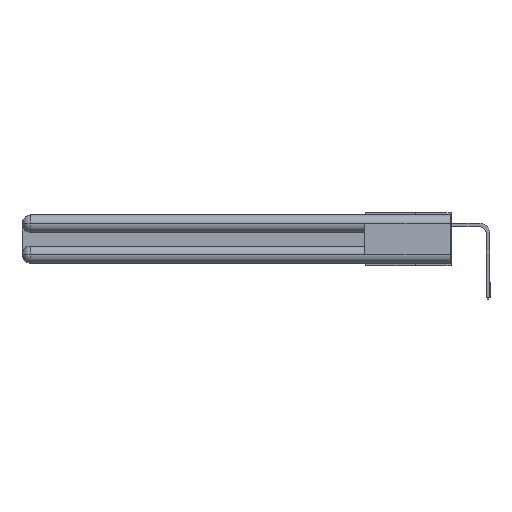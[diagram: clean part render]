
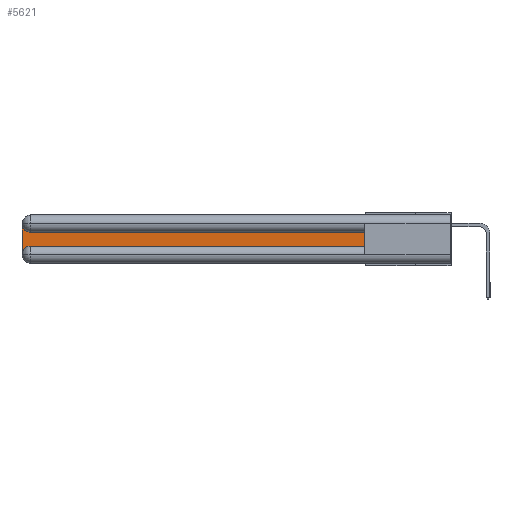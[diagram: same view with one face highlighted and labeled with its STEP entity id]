
A CAD part, left-side view. The second image highlights one B-rep face of the part: STEP entity #5621.
In plain terms, the highlighted planar face has unit normal (-1, 0, 0).
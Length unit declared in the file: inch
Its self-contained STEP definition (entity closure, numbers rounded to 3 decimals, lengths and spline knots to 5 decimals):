
#64 = LINE ( 'NONE', #15927, #16240 ) ;
#335 = CARTESIAN_POINT ( 'NONE',  ( 0.075, 0.6, -0.2175 ) ) ;
#463 = CARTESIAN_POINT ( 'NONE',  ( 0.075, 2.94, -0.2775 ) ) ;
#1160 = VECTOR ( 'NONE', #6062, 39.37008 ) ;
#1681 = CARTESIAN_POINT ( 'NONE',  ( 0.075, 2.94, -0.1225 ) ) ;
#4650 = AXIS2_PLACEMENT_3D ( 'NONE', #8963, #23938, #19724 ) ;
#4861 = VERTEX_POINT ( 'NONE', #23996 ) ;
#4953 = ORIENTED_EDGE ( 'NONE', *, *, #12622, .T. ) ;
#5380 = DIRECTION ( 'NONE',  ( 0., 1., 0. ) ) ;
#5621 = ADVANCED_FACE ( 'NONE', ( #23289 ), #14612, .F. ) ;
#5836 = VECTOR ( 'NONE', #11430, 39.37008 ) ;
#6042 = DIRECTION ( 'NONE',  ( 1., 0., 0. ) ) ;
#6062 = DIRECTION ( 'NONE',  ( 0., 0., 1. ) ) ;
#6643 = EDGE_CURVE ( 'NONE', #27674, #13125, #64, .T. ) ;
#6910 = ORIENTED_EDGE ( 'NONE', *, *, #27615, .T. ) ;
#7510 = ORIENTED_EDGE ( 'NONE', *, *, #6643, .T. ) ;
#8207 = AXIS2_PLACEMENT_3D ( 'NONE', #463, #11471, #17662 ) ;
#8359 = CIRCLE ( 'NONE', #8207, 0.06 ) ;
#8844 = CIRCLE ( 'NONE', #4650, 0.06 ) ;
#8963 = CARTESIAN_POINT ( 'NONE',  ( 0.075, 2.94, -0.0625 ) ) ;
#11143 = CARTESIAN_POINT ( 'NONE',  ( 0.075, 0.6, -0.1225 ) ) ;
#11430 = DIRECTION ( 'NONE',  ( 0., -1., 0. ) ) ;
#11471 = DIRECTION ( 'NONE',  ( 1., 0., 0. ) ) ;
#12327 = ORIENTED_EDGE ( 'NONE', *, *, #13479, .T. ) ;
#12622 = EDGE_CURVE ( 'NONE', #26845, #27674, #16632, .T. ) ;
#13125 = VERTEX_POINT ( 'NONE', #1681 ) ;
#13479 = EDGE_CURVE ( 'NONE', #13125, #24342, #8844, .T. ) ;
#14219 = CARTESIAN_POINT ( 'NONE',  ( 0.075, 3., -0.0625 ) ) ;
#14586 = CARTESIAN_POINT ( 'NONE',  ( 0.075, 2.94, -0.2175 ) ) ;
#14612 = PLANE ( 'NONE',  #21056 ) ;
#14716 = VECTOR ( 'NONE', #23486, 39.37008 ) ;
#14966 = CARTESIAN_POINT ( 'NONE',  ( 0.075, 3., -0.1225 ) ) ;
#15616 = LINE ( 'NONE', #335, #5836 ) ;
#15674 = CARTESIAN_POINT ( 'NONE',  ( 0.075, 0.6, -0.2175 ) ) ;
#15927 = CARTESIAN_POINT ( 'NONE',  ( 0.075, 0.6, -0.1225 ) ) ;
#16240 = VECTOR ( 'NONE', #5380, 39.37008 ) ;
#16632 = LINE ( 'NONE', #23283, #1160 ) ;
#17538 = ORIENTED_EDGE ( 'NONE', *, *, #25268, .T. ) ;
#17662 = DIRECTION ( 'NONE',  ( 0., 0., -1. ) ) ;
#19724 = DIRECTION ( 'NONE',  ( 0., 0., -1. ) ) ;
#20723 = LINE ( 'NONE', #25642, #14716 ) ;
#20839 = EDGE_CURVE ( 'NONE', #4861, #24428, #8359, .T. ) ;
#21043 = DIRECTION ( 'NONE',  ( 0., 0., -1. ) ) ;
#21056 = AXIS2_PLACEMENT_3D ( 'NONE', #14966, #6042, #21043 ) ;
#23283 = CARTESIAN_POINT ( 'NONE',  ( 0.075, 0.6, -0.2175 ) ) ;
#23289 = FACE_OUTER_BOUND ( 'NONE', #26970, .T. ) ;
#23486 = DIRECTION ( 'NONE',  ( 0., 0., -1. ) ) ;
#23938 = DIRECTION ( 'NONE',  ( 1., 0., 0. ) ) ;
#23996 = CARTESIAN_POINT ( 'NONE',  ( 0.075, 3., -0.2775 ) ) ;
#24342 = VERTEX_POINT ( 'NONE', #14219 ) ;
#24428 = VERTEX_POINT ( 'NONE', #14586 ) ;
#25268 = EDGE_CURVE ( 'NONE', #24342, #4861, #20723, .T. ) ;
#25642 = CARTESIAN_POINT ( 'NONE',  ( 0.075, 3., -0.2175 ) ) ;
#26034 = ORIENTED_EDGE ( 'NONE', *, *, #20839, .T. ) ;
#26845 = VERTEX_POINT ( 'NONE', #15674 ) ;
#26970 = EDGE_LOOP ( 'NONE', ( #7510, #12327, #17538, #26034, #6910, #4953 ) ) ;
#27615 = EDGE_CURVE ( 'NONE', #24428, #26845, #15616, .T. ) ;
#27674 = VERTEX_POINT ( 'NONE', #11143 ) ;
